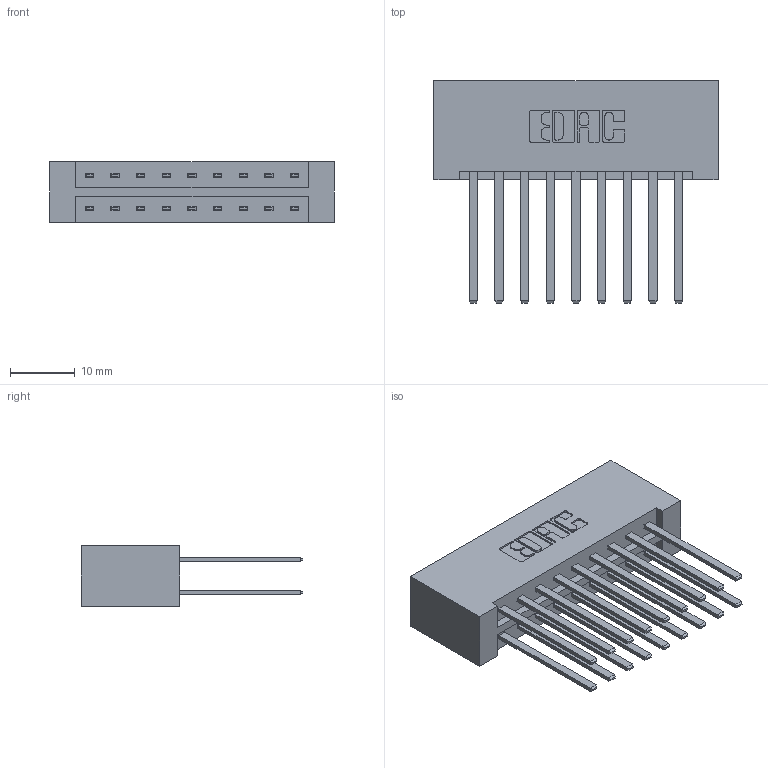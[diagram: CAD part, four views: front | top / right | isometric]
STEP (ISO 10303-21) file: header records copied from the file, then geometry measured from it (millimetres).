
FILE_DESCRIPTION (( 'STEP AP203' ), '1' );
FILE_NAME ('333-018-544-201.STEP', '2019-08-09T13:46:13', ( '' ), ( '' ), 'SwSTEP 2.0', 'SolidWorks 2016', '' );
FILE_SCHEMA (( 'CONFIG_CONTROL_DESIGN' ));
Length unit declared in the file: inch
Products named in the file (3): 345-292-001_345-293-144; 333 Part_Lugless; 333-018-544-201
Assembly tree (19 placements, depth 2):
  333-018-544-201
    333 Part_Lugless
    345-292-001_345-293-144  x18
Bounding box: 43.92 x 34.3 x 9.4 mm (x, y, z)
Volume: 5059.6 mm3; surface area: 6463.9 mm2
Topology: 19 solids, 19 shells, 934 faces, 2753 edges, 1810 vertices
Faces by surface type: plane 642, cylinder 292
Entity records: 9597 total; most frequent: CARTESIAN_POINT 1626, ORIENTED_EDGE 1562, DIRECTION 1437, EDGE_CURVE 781, LINE 665, VECTOR 665, VERTEX_POINT 518, AXIS2_PLACEMENT_3D 386
